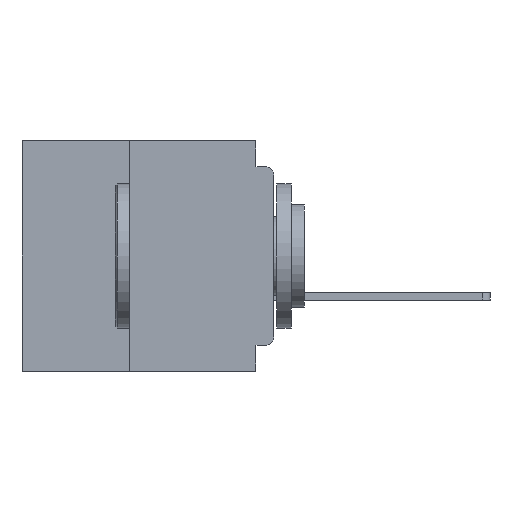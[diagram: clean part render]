
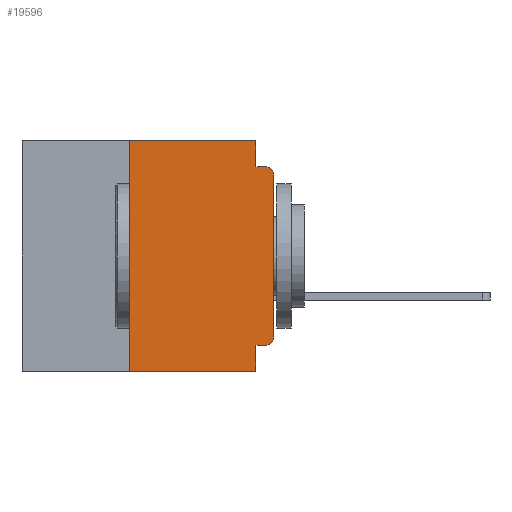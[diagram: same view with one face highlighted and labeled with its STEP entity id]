
A CAD part, left-side view. The second image highlights one B-rep face of the part: STEP entity #19596.
In plain terms, the highlighted planar face has unit normal (-1, 0, 0).
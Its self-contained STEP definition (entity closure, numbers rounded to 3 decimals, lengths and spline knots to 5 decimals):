
#710 = EDGE_CURVE ( 'NONE', #11870, #7070, #44058, .T. ) ;
#2382 = CARTESIAN_POINT ( 'NONE',  ( 0., 0.031, -0.4 ) ) ;
#2564 = CARTESIAN_POINT ( 'NONE',  ( 0., 0., -0.355 ) ) ;
#3625 = LINE ( 'NONE', #43462, #13764 ) ;
#5230 = EDGE_CURVE ( 'NONE', #27231, #7070, #43527, .T. ) ;
#5294 = CARTESIAN_POINT ( 'NONE',  ( 0., 0.031, -0.355 ) ) ;
#5440 = ORIENTED_EDGE ( 'NONE', *, *, #32714, .T. ) ;
#6194 = ORIENTED_EDGE ( 'NONE', *, *, #39997, .F. ) ;
#6501 = EDGE_CURVE ( 'NONE', #38184, #27231, #34895, .T. ) ;
#6798 = CARTESIAN_POINT ( 'NONE',  ( 0., 0.015, -0.34 ) ) ;
#7070 = VERTEX_POINT ( 'NONE', #27621 ) ;
#7710 = CARTESIAN_POINT ( 'NONE',  ( 0., 0., -0.06 ) ) ;
#8061 = DIRECTION ( 'NONE',  ( 1., 0., 0. ) ) ;
#8908 = ORIENTED_EDGE ( 'NONE', *, *, #6501, .F. ) ;
#9777 = VERTEX_POINT ( 'NONE', #14822 ) ;
#11783 = DIRECTION ( 'NONE',  ( 0., 0., -1. ) ) ;
#11870 = VERTEX_POINT ( 'NONE', #7710 ) ;
#12090 = CARTESIAN_POINT ( 'NONE',  ( 0., 0.031, 0. ) ) ;
#12592 = EDGE_CURVE ( 'NONE', #36025, #11870, #58307, .T. ) ;
#13764 = VECTOR ( 'NONE', #18730, 39.37008 ) ;
#14538 = DIRECTION ( 'NONE',  ( 0., 0., -1. ) ) ;
#14666 = DIRECTION ( 'NONE',  ( -1., 0., 0. ) ) ;
#14726 = CARTESIAN_POINT ( 'NONE',  ( 0., 0.015, -0.355 ) ) ;
#14760 = CARTESIAN_POINT ( 'NONE',  ( 0., 0.015, -0.06 ) ) ;
#14822 = CARTESIAN_POINT ( 'NONE',  ( 0., 0.25, 0. ) ) ;
#15627 = DIRECTION ( 'NONE',  ( 0., -1., 0. ) ) ;
#15659 = LINE ( 'NONE', #2564, #53538 ) ;
#16760 = VECTOR ( 'NONE', #22191, 39.37008 ) ;
#16940 = VECTOR ( 'NONE', #33166, 39.37008 ) ;
#17067 = EDGE_CURVE ( 'NONE', #28663, #36025, #19944, .T. ) ;
#17574 = DIRECTION ( 'NONE',  ( 0., 1., 0. ) ) ;
#17628 = CARTESIAN_POINT ( 'NONE',  ( 0., 0.437, 0. ) ) ;
#17695 = CARTESIAN_POINT ( 'NONE',  ( 0., 0.031, 0. ) ) ;
#17857 = CARTESIAN_POINT ( 'NONE',  ( 0., 0.031, -0.045 ) ) ;
#18328 = LINE ( 'NONE', #2382, #16760 ) ;
#18730 = DIRECTION ( 'NONE',  ( 0., 0., 1. ) ) ;
#19596 = ADVANCED_FACE ( 'NONE', ( #45977 ), #32886, .F. ) ;
#19862 = ORIENTED_EDGE ( 'NONE', *, *, #21867, .F. ) ;
#19944 = CIRCLE ( 'NONE', #61036, 0.015 ) ;
#21867 = EDGE_CURVE ( 'NONE', #9777, #38184, #24744, .T. ) ;
#22191 = DIRECTION ( 'NONE',  ( 0., 0., -1. ) ) ;
#23523 = CARTESIAN_POINT ( 'NONE',  ( 0., 0., 0. ) ) ;
#24043 = CARTESIAN_POINT ( 'NONE',  ( 0., 0.031, -0.4 ) ) ;
#24395 = CARTESIAN_POINT ( 'NONE',  ( 0., 0.437, 0. ) ) ;
#24744 = LINE ( 'NONE', #24395, #62455 ) ;
#26077 = LINE ( 'NONE', #54928, #37704 ) ;
#26441 = CARTESIAN_POINT ( 'NONE',  ( 0., 0., -0.045 ) ) ;
#26795 = AXIS2_PLACEMENT_3D ( 'NONE', #17628, #8061, #42817 ) ;
#27231 = VERTEX_POINT ( 'NONE', #17857 ) ;
#27621 = CARTESIAN_POINT ( 'NONE',  ( 0., 0.015, -0.045 ) ) ;
#27804 = ORIENTED_EDGE ( 'NONE', *, *, #55872, .F. ) ;
#28501 = DIRECTION ( 'NONE',  ( 0., 0., 1. ) ) ;
#28663 = VERTEX_POINT ( 'NONE', #14726 ) ;
#31137 = VERTEX_POINT ( 'NONE', #5294 ) ;
#31385 = ORIENTED_EDGE ( 'NONE', *, *, #53141, .F. ) ;
#32714 = EDGE_CURVE ( 'NONE', #54520, #38426, #26077, .T. ) ;
#32886 = PLANE ( 'NONE',  #26795 ) ;
#33166 = DIRECTION ( 'NONE',  ( 0., 0., -1. ) ) ;
#34895 = LINE ( 'NONE', #17695, #16940 ) ;
#35607 = CARTESIAN_POINT ( 'NONE',  ( 0., 0.25, -0.4 ) ) ;
#36025 = VERTEX_POINT ( 'NONE', #61070 ) ;
#37512 = ORIENTED_EDGE ( 'NONE', *, *, #5230, .F. ) ;
#37704 = VECTOR ( 'NONE', #15627, 39.37008 ) ;
#38184 = VERTEX_POINT ( 'NONE', #12090 ) ;
#38426 = VERTEX_POINT ( 'NONE', #24043 ) ;
#39810 = ORIENTED_EDGE ( 'NONE', *, *, #12592, .T. ) ;
#39997 = EDGE_CURVE ( 'NONE', #31137, #38426, #18328, .T. ) ;
#41576 = DIRECTION ( 'NONE',  ( -1., 0., 0. ) ) ;
#42817 = DIRECTION ( 'NONE',  ( 0., 0., -1. ) ) ;
#43462 = CARTESIAN_POINT ( 'NONE',  ( 0., 0.25, -0.4 ) ) ;
#43527 = LINE ( 'NONE', #26441, #54977 ) ;
#43774 = VECTOR ( 'NONE', #28501, 39.37008 ) ;
#44058 = CIRCLE ( 'NONE', #53485, 0.015 ) ;
#44098 = DIRECTION ( 'NONE',  ( 0., -1., 0. ) ) ;
#45977 = FACE_OUTER_BOUND ( 'NONE', #53059, .T. ) ;
#46083 = ORIENTED_EDGE ( 'NONE', *, *, #710, .T. ) ;
#46132 = DIRECTION ( 'NONE',  ( 0., -1., 0. ) ) ;
#53059 = EDGE_LOOP ( 'NONE', ( #39810, #46083, #37512, #8908, #19862, #31385, #5440, #6194, #27804, #64071 ) ) ;
#53141 = EDGE_CURVE ( 'NONE', #54520, #9777, #3625, .T. ) ;
#53485 = AXIS2_PLACEMENT_3D ( 'NONE', #14760, #14666, #14538 ) ;
#53538 = VECTOR ( 'NONE', #17574, 39.37008 ) ;
#54520 = VERTEX_POINT ( 'NONE', #35607 ) ;
#54928 = CARTESIAN_POINT ( 'NONE',  ( 0., 0.437, -0.4 ) ) ;
#54977 = VECTOR ( 'NONE', #46132, 39.37008 ) ;
#55872 = EDGE_CURVE ( 'NONE', #28663, #31137, #15659, .T. ) ;
#58307 = LINE ( 'NONE', #23523, #43774 ) ;
#61036 = AXIS2_PLACEMENT_3D ( 'NONE', #6798, #41576, #11783 ) ;
#61070 = CARTESIAN_POINT ( 'NONE',  ( 0., 0., -0.34 ) ) ;
#62455 = VECTOR ( 'NONE', #44098, 39.37008 ) ;
#64071 = ORIENTED_EDGE ( 'NONE', *, *, #17067, .T. ) ;
